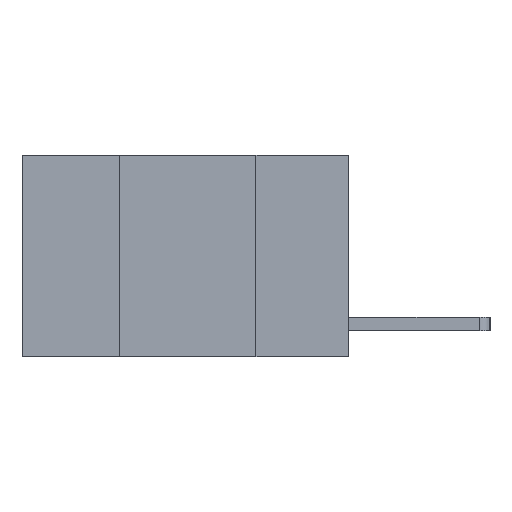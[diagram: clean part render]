
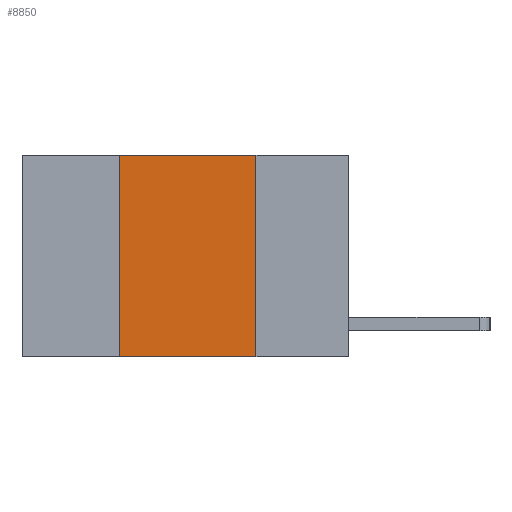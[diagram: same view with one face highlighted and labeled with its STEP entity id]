
A CAD part, left-side view. The second image highlights one B-rep face of the part: STEP entity #8850.
In plain terms, the highlighted planar face has unit normal (-1, 0, 0).
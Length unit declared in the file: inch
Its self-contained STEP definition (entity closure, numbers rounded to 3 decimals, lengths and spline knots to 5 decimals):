
#13 = VECTOR ( 'NONE', #2828, 39.37008 ) ;
#206 = VERTEX_POINT ( 'NONE', #6774 ) ;
#238 = LINE ( 'NONE', #8178, #13 ) ;
#249 = CARTESIAN_POINT ( 'NONE',  ( 0., 0.42, 0. ) ) ;
#1126 = CARTESIAN_POINT ( 'NONE',  ( 0., 0.17, 0. ) ) ;
#1520 = DIRECTION ( 'NONE',  ( 0., 0., 1. ) ) ;
#1770 = PLANE ( 'NONE',  #7963 ) ;
#1967 = DIRECTION ( 'NONE',  ( 0., 0., -1. ) ) ;
#2171 = EDGE_LOOP ( 'NONE', ( #3997, #5342, #6994, #8064 ) ) ;
#2740 = VECTOR ( 'NONE', #4407, 39.37008 ) ;
#2828 = DIRECTION ( 'NONE',  ( 0., -1., 0. ) ) ;
#2941 = LINE ( 'NONE', #6565, #6796 ) ;
#2971 = VERTEX_POINT ( 'NONE', #249 ) ;
#3196 = CARTESIAN_POINT ( 'NONE',  ( 0., 0.42, -0.37 ) ) ;
#3288 = DIRECTION ( 'NONE',  ( 0., 0., -1. ) ) ;
#3997 = ORIENTED_EDGE ( 'NONE', *, *, #7376, .F. ) ;
#4407 = DIRECTION ( 'NONE',  ( 0., -1., 0. ) ) ;
#4409 = EDGE_CURVE ( 'NONE', #5188, #206, #4782, .T. ) ;
#4651 = VECTOR ( 'NONE', #1520, 39.37008 ) ;
#4782 = LINE ( 'NONE', #6685, #2740 ) ;
#5188 = VERTEX_POINT ( 'NONE', #3196 ) ;
#5342 = ORIENTED_EDGE ( 'NONE', *, *, #8972, .F. ) ;
#6128 = CARTESIAN_POINT ( 'NONE',  ( 0., 0.42, 0. ) ) ;
#6565 = CARTESIAN_POINT ( 'NONE',  ( 0., 0.17, 0. ) ) ;
#6685 = CARTESIAN_POINT ( 'NONE',  ( 0., 0.6, -0.37 ) ) ;
#6774 = CARTESIAN_POINT ( 'NONE',  ( 0., 0.17, -0.37 ) ) ;
#6796 = VECTOR ( 'NONE', #1967, 39.37008 ) ;
#6994 = ORIENTED_EDGE ( 'NONE', *, *, #9152, .F. ) ;
#7113 = CARTESIAN_POINT ( 'NONE',  ( 0., 0.6, 0. ) ) ;
#7330 = VERTEX_POINT ( 'NONE', #1126 ) ;
#7376 = EDGE_CURVE ( 'NONE', #7330, #206, #2941, .T. ) ;
#7597 = FACE_OUTER_BOUND ( 'NONE', #2171, .T. ) ;
#7880 = DIRECTION ( 'NONE',  ( 1., 0., 0. ) ) ;
#7963 = AXIS2_PLACEMENT_3D ( 'NONE', #7113, #7880, #3288 ) ;
#8064 = ORIENTED_EDGE ( 'NONE', *, *, #4409, .T. ) ;
#8178 = CARTESIAN_POINT ( 'NONE',  ( 0., 0.6, 0. ) ) ;
#8234 = LINE ( 'NONE', #6128, #4651 ) ;
#8850 = ADVANCED_FACE ( 'NONE', ( #7597 ), #1770, .F. ) ;
#8972 = EDGE_CURVE ( 'NONE', #2971, #7330, #238, .T. ) ;
#9152 = EDGE_CURVE ( 'NONE', #5188, #2971, #8234, .T. ) ;
